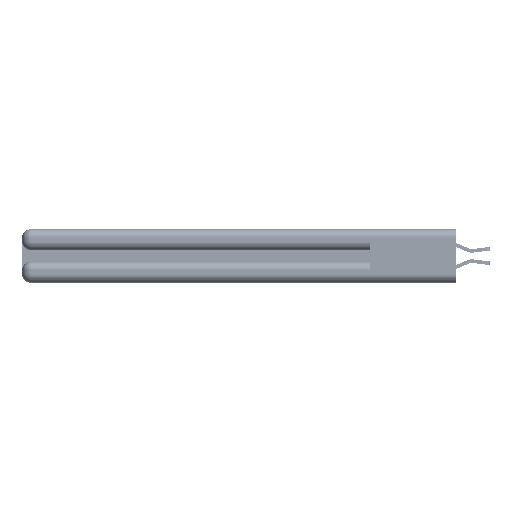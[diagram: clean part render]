
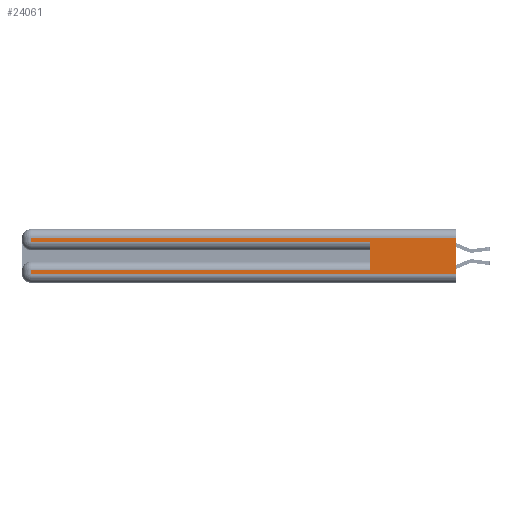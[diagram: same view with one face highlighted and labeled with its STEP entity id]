
A CAD part, left-side view. The second image highlights one B-rep face of the part: STEP entity #24061.
In plain terms, the highlighted planar face has unit normal (-1, 0, 0).
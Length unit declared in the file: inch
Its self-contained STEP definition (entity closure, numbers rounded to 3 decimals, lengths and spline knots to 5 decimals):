
#170 = CARTESIAN_POINT ( 'NONE',  ( 0., 0., 0.285 ) ) ;
#596 = CARTESIAN_POINT ( 'NONE',  ( 0., 0., 0.06 ) ) ;
#1379 = VECTOR ( 'NONE', #3844, 39.37008 ) ;
#1747 = EDGE_LOOP ( 'NONE', ( #5377, #22140, #19049, #33892, #11742, #8119, #39943, #12415 ) ) ;
#2380 = CARTESIAN_POINT ( 'NONE',  ( 0., 0.6, 0.085 ) ) ;
#3278 = EDGE_CURVE ( 'NONE', #14864, #6536, #28258, .T. ) ;
#3536 = VECTOR ( 'NONE', #5067, 39.37008 ) ;
#3844 = DIRECTION ( 'NONE',  ( 0., 0., -1. ) ) ;
#5044 = VERTEX_POINT ( 'NONE', #2380 ) ;
#5067 = DIRECTION ( 'NONE',  ( 0., 0., 1. ) ) ;
#5377 = ORIENTED_EDGE ( 'NONE', *, *, #52348, .F. ) ;
#6118 = DIRECTION ( 'NONE',  ( 1., 0., 0. ) ) ;
#6216 = CARTESIAN_POINT ( 'NONE',  ( 0., 0., 0.31 ) ) ;
#6536 = VERTEX_POINT ( 'NONE', #31158 ) ;
#7952 = DIRECTION ( 'NONE',  ( 0., 1., 0. ) ) ;
#7962 = CARTESIAN_POINT ( 'NONE',  ( 0., 0., 0.06 ) ) ;
#8119 = ORIENTED_EDGE ( 'NONE', *, *, #37982, .T. ) ;
#8155 = DIRECTION ( 'NONE',  ( 0., -1., 0. ) ) ;
#8596 = DIRECTION ( 'NONE',  ( 0., -1., 0. ) ) ;
#9592 = VERTEX_POINT ( 'NONE', #35456 ) ;
#10134 = VERTEX_POINT ( 'NONE', #14022 ) ;
#10310 = DIRECTION ( 'NONE',  ( 0., 0., -1. ) ) ;
#10521 = LINE ( 'NONE', #170, #39869 ) ;
#10573 = LINE ( 'NONE', #28829, #1379 ) ;
#10684 = VECTOR ( 'NONE', #7952, 39.37008 ) ;
#10849 = CARTESIAN_POINT ( 'NONE',  ( 0., 0., 0.37 ) ) ;
#11742 = ORIENTED_EDGE ( 'NONE', *, *, #37640, .F. ) ;
#12415 = ORIENTED_EDGE ( 'NONE', *, *, #23677, .T. ) ;
#13292 = FACE_OUTER_BOUND ( 'NONE', #1747, .T. ) ;
#14022 = CARTESIAN_POINT ( 'NONE',  ( 0., 2.94, 0.085 ) ) ;
#14216 = CARTESIAN_POINT ( 'NONE',  ( 0., 0.6, 0.145 ) ) ;
#14312 = LINE ( 'NONE', #49017, #23463 ) ;
#14864 = VERTEX_POINT ( 'NONE', #36269 ) ;
#17927 = VECTOR ( 'NONE', #8155, 39.37008 ) ;
#19049 = ORIENTED_EDGE ( 'NONE', *, *, #30433, .T. ) ;
#19811 = VECTOR ( 'NONE', #22470, 39.37008 ) ;
#20563 = DIRECTION ( 'NONE',  ( 0., 0., -1. ) ) ;
#21790 = LINE ( 'NONE', #49563, #10684 ) ;
#22140 = ORIENTED_EDGE ( 'NONE', *, *, #3278, .T. ) ;
#22470 = DIRECTION ( 'NONE',  ( 0., 1., 0. ) ) ;
#23463 = VECTOR ( 'NONE', #48833, 39.37008 ) ;
#23602 = CARTESIAN_POINT ( 'NONE',  ( 0., 2.94, 0.285 ) ) ;
#23677 = EDGE_CURVE ( 'NONE', #33028, #46810, #31601, .T. ) ;
#24061 = ADVANCED_FACE ( 'NONE', ( #13292 ), #30194, .F. ) ;
#28258 = LINE ( 'NONE', #6216, #19811 ) ;
#28829 = CARTESIAN_POINT ( 'NONE',  ( 0., 2.94, 0.37 ) ) ;
#30194 = PLANE ( 'NONE',  #53764 ) ;
#30433 = EDGE_CURVE ( 'NONE', #6536, #46956, #14312, .T. ) ;
#31158 = CARTESIAN_POINT ( 'NONE',  ( 0., 2.94, 0.31 ) ) ;
#31601 = LINE ( 'NONE', #7962, #17927 ) ;
#33028 = VERTEX_POINT ( 'NONE', #53283 ) ;
#33501 = VECTOR ( 'NONE', #20563, 39.37008 ) ;
#33892 = ORIENTED_EDGE ( 'NONE', *, *, #43983, .T. ) ;
#35456 = CARTESIAN_POINT ( 'NONE',  ( 0., 0.6, 0.285 ) ) ;
#36269 = CARTESIAN_POINT ( 'NONE',  ( 0., 0., 0.31 ) ) ;
#37640 = EDGE_CURVE ( 'NONE', #5044, #9592, #47976, .T. ) ;
#37982 = EDGE_CURVE ( 'NONE', #5044, #10134, #21790, .T. ) ;
#39869 = VECTOR ( 'NONE', #8596, 39.37008 ) ;
#39943 = ORIENTED_EDGE ( 'NONE', *, *, #43826, .T. ) ;
#43826 = EDGE_CURVE ( 'NONE', #10134, #33028, #10573, .T. ) ;
#43983 = EDGE_CURVE ( 'NONE', #46956, #9592, #10521, .T. ) ;
#45516 = CARTESIAN_POINT ( 'NONE',  ( 0., 0., 0.37 ) ) ;
#46810 = VERTEX_POINT ( 'NONE', #596 ) ;
#46956 = VERTEX_POINT ( 'NONE', #23602 ) ;
#47976 = LINE ( 'NONE', #14216, #3536 ) ;
#48833 = DIRECTION ( 'NONE',  ( 0., 0., -1. ) ) ;
#49017 = CARTESIAN_POINT ( 'NONE',  ( 0., 2.94, 0.37 ) ) ;
#49563 = CARTESIAN_POINT ( 'NONE',  ( 0., 0., 0.085 ) ) ;
#51809 = LINE ( 'NONE', #45516, #33501 ) ;
#52348 = EDGE_CURVE ( 'NONE', #14864, #46810, #51809, .T. ) ;
#53283 = CARTESIAN_POINT ( 'NONE',  ( 0., 2.94, 0.06 ) ) ;
#53764 = AXIS2_PLACEMENT_3D ( 'NONE', #10849, #6118, #10310 ) ;
